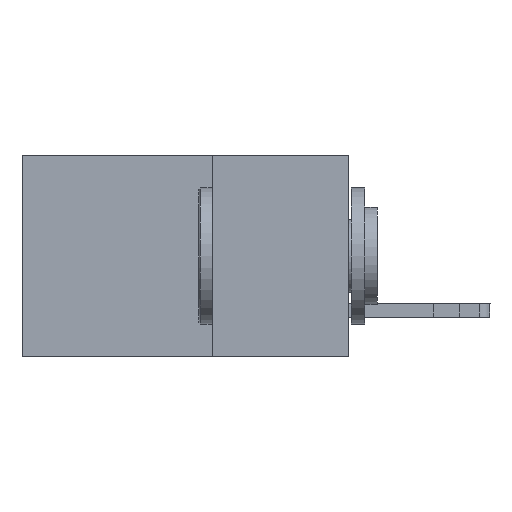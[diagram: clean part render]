
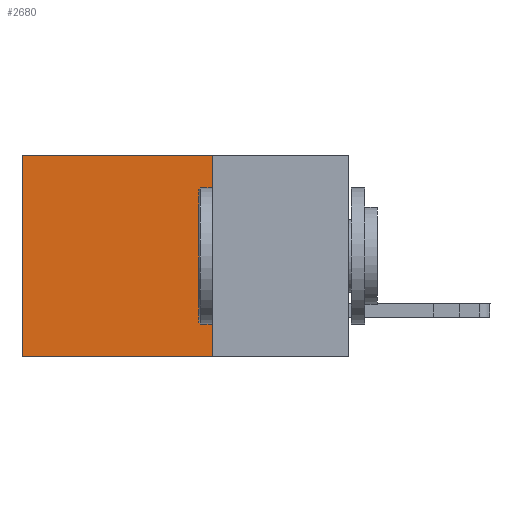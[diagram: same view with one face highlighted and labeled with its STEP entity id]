
A CAD part, left-side view. The second image highlights one B-rep face of the part: STEP entity #2680.
In plain terms, the highlighted planar face has unit normal (-1, 0, 0).
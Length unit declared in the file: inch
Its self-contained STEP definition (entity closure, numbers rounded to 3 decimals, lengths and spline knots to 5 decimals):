
#143 = CARTESIAN_POINT ( 'NONE',  ( 0.2615, 0.25, -0.37 ) ) ;
#194 = LINE ( 'NONE', #8134, #12190 ) ;
#273 = DIRECTION ( 'NONE',  ( 0., 1., 0. ) ) ;
#389 = CARTESIAN_POINT ( 'NONE',  ( 0.2615, 0.25, 0. ) ) ;
#694 = PLANE ( 'NONE',  #8097 ) ;
#731 = EDGE_CURVE ( 'NONE', #7751, #8283, #10072, .T. ) ;
#815 = CARTESIAN_POINT ( 'NONE',  ( 0.2615, 0.25, -0.37 ) ) ;
#1377 = VECTOR ( 'NONE', #3015, 39.37008 ) ;
#1969 = DIRECTION ( 'NONE',  ( 0., 0., -1. ) ) ;
#2680 = ADVANCED_FACE ( 'NONE', ( #5304 ), #694, .F. ) ;
#2699 = DIRECTION ( 'NONE',  ( 0., 1., 0. ) ) ;
#3015 = DIRECTION ( 'NONE',  ( 0., 0., -1. ) ) ;
#3026 = CARTESIAN_POINT ( 'NONE',  ( 0.2615, 0.25, 0. ) ) ;
#3067 = CARTESIAN_POINT ( 'NONE',  ( 0.2615, 0.6, -0.37 ) ) ;
#3758 = LINE ( 'NONE', #389, #5974 ) ;
#4058 = EDGE_CURVE ( 'NONE', #5856, #7751, #194, .T. ) ;
#4654 = EDGE_CURVE ( 'NONE', #5605, #8283, #8993, .T. ) ;
#4734 = EDGE_CURVE ( 'NONE', #5856, #5605, #3758, .T. ) ;
#5004 = ORIENTED_EDGE ( 'NONE', *, *, #731, .F. ) ;
#5205 = VECTOR ( 'NONE', #2699, 39.37008 ) ;
#5304 = FACE_OUTER_BOUND ( 'NONE', #9032, .T. ) ;
#5605 = VERTEX_POINT ( 'NONE', #8448 ) ;
#5856 = VERTEX_POINT ( 'NONE', #3026 ) ;
#5974 = VECTOR ( 'NONE', #273, 39.37008 ) ;
#7751 = VERTEX_POINT ( 'NONE', #143 ) ;
#8097 = AXIS2_PLACEMENT_3D ( 'NONE', #815, #8253, #1969 ) ;
#8134 = CARTESIAN_POINT ( 'NONE',  ( 0.2615, 0.25, -0.37 ) ) ;
#8253 = DIRECTION ( 'NONE',  ( 1., 0., 0. ) ) ;
#8283 = VERTEX_POINT ( 'NONE', #3067 ) ;
#8412 = DIRECTION ( 'NONE',  ( 0., 0., -1. ) ) ;
#8448 = CARTESIAN_POINT ( 'NONE',  ( 0.2615, 0.6, 0. ) ) ;
#8549 = CARTESIAN_POINT ( 'NONE',  ( 0.2615, 0.6, -0.37 ) ) ;
#8993 = LINE ( 'NONE', #8549, #1377 ) ;
#9032 = EDGE_LOOP ( 'NONE', ( #9812, #5004, #10403, #10636 ) ) ;
#9812 = ORIENTED_EDGE ( 'NONE', *, *, #4654, .T. ) ;
#10072 = LINE ( 'NONE', #11435, #5205 ) ;
#10403 = ORIENTED_EDGE ( 'NONE', *, *, #4058, .F. ) ;
#10636 = ORIENTED_EDGE ( 'NONE', *, *, #4734, .T. ) ;
#11435 = CARTESIAN_POINT ( 'NONE',  ( 0.2615, 0.25, -0.37 ) ) ;
#12190 = VECTOR ( 'NONE', #8412, 39.37008 ) ;
